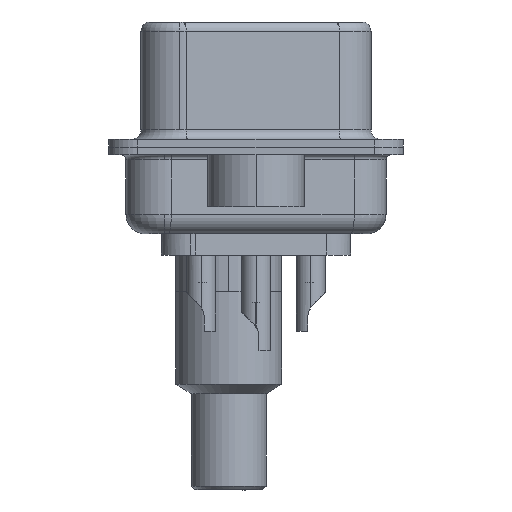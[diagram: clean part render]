
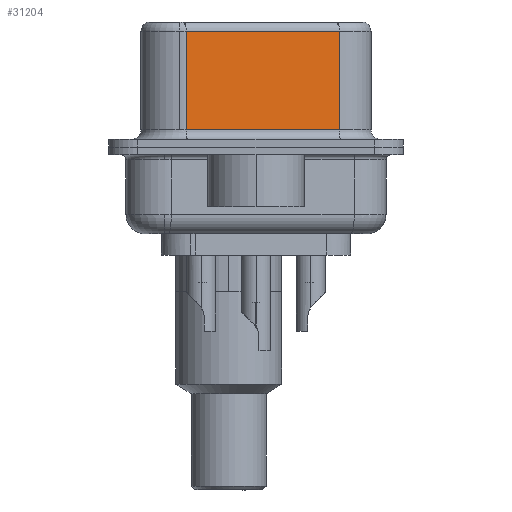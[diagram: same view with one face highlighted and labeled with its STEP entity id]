
A CAD part, left-side view. The second image highlights one B-rep face of the part: STEP entity #31204.
In plain terms, the highlighted planar face has unit normal (-0.985, -0.174, 0).
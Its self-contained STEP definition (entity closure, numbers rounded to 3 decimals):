
#564 = CARTESIAN_POINT ( 'NONE',  ( 5.132, -4.322, 6.02 ) ) ;
#2629 = EDGE_CURVE ( 'NONE', #15933, #23288, #30191, .T. ) ;
#2773 = ORIENTED_EDGE ( 'NONE', *, *, #27200, .T. ) ;
#3308 = VERTEX_POINT ( 'NONE', #17493 ) ;
#3505 = CARTESIAN_POINT ( 'NONE',  ( 5.132, -4.322, 6.02 ) ) ;
#3775 = DIRECTION ( 'NONE',  ( 0.985, 0.174, 0. ) ) ;
#4037 = ORIENTED_EDGE ( 'NONE', *, *, #2629, .F. ) ;
#4174 = VECTOR ( 'NONE', #15285, 1000. ) ;
#6143 = CARTESIAN_POINT ( 'NONE',  ( 5.132, -4.322, 6.52 ) ) ;
#6882 = VERTEX_POINT ( 'NONE', #31883 ) ;
#7245 = CARTESIAN_POINT ( 'NONE',  ( 3.73, 3.628, 6.52 ) ) ;
#7365 = DIRECTION ( 'NONE',  ( 0., 0., -1. ) ) ;
#8212 = DIRECTION ( 'NONE',  ( 0., 0., -1. ) ) ;
#8989 = ORIENTED_EDGE ( 'NONE', *, *, #9594, .T. ) ;
#9594 = EDGE_CURVE ( 'NONE', #3308, #23288, #29544, .T. ) ;
#9803 = DIRECTION ( 'NONE',  ( 0.174, -0.985, 0. ) ) ;
#10433 = LINE ( 'NONE', #7245, #29518 ) ;
#10443 = ORIENTED_EDGE ( 'NONE', *, *, #25350, .T. ) ;
#12739 = FACE_OUTER_BOUND ( 'NONE', #14505, .T. ) ;
#14505 = EDGE_LOOP ( 'NONE', ( #4037, #2773, #10443, #8989 ) ) ;
#15285 = DIRECTION ( 'NONE',  ( -0.174, 0.985, 0. ) ) ;
#15933 = VERTEX_POINT ( 'NONE', #3505 ) ;
#16032 = PLANE ( 'NONE',  #27420 ) ;
#16471 = LINE ( 'NONE', #564, #4174 ) ;
#17493 = CARTESIAN_POINT ( 'NONE',  ( 3.73, 3.628, 0.9 ) ) ;
#21002 = DIRECTION ( 'NONE',  ( -0.174, 0.985, 0. ) ) ;
#22872 = VECTOR ( 'NONE', #9803, 1000. ) ;
#23288 = VERTEX_POINT ( 'NONE', #30153 ) ;
#23520 = VECTOR ( 'NONE', #8212, 1000. ) ;
#25350 = EDGE_CURVE ( 'NONE', #6882, #3308, #10433, .T. ) ;
#27192 = CARTESIAN_POINT ( 'NONE',  ( 5.132, -4.322, 0.9 ) ) ;
#27200 = EDGE_CURVE ( 'NONE', #15933, #6882, #16471, .T. ) ;
#27420 = AXIS2_PLACEMENT_3D ( 'NONE', #6143, #3775, #21002 ) ;
#28978 = CARTESIAN_POINT ( 'NONE',  ( 5.132, -4.322, 6.52 ) ) ;
#29518 = VECTOR ( 'NONE', #7365, 1000. ) ;
#29544 = LINE ( 'NONE', #27192, #22872 ) ;
#30153 = CARTESIAN_POINT ( 'NONE',  ( 5.132, -4.322, 0.9 ) ) ;
#30191 = LINE ( 'NONE', #28978, #23520 ) ;
#31204 = ADVANCED_FACE ( 'NONE', ( #12739 ), #16032, .F. ) ;
#31883 = CARTESIAN_POINT ( 'NONE',  ( 3.73, 3.628, 6.02 ) ) ;
